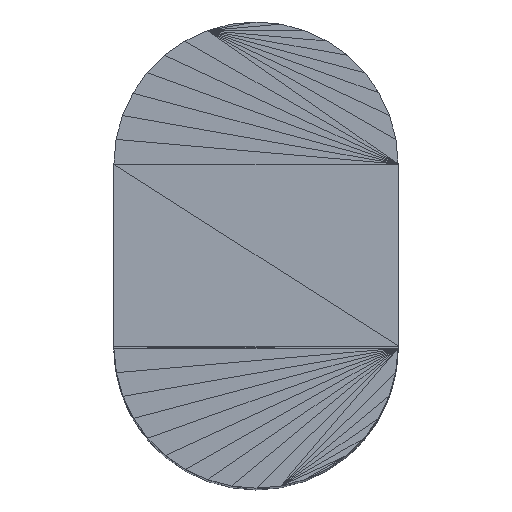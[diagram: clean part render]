
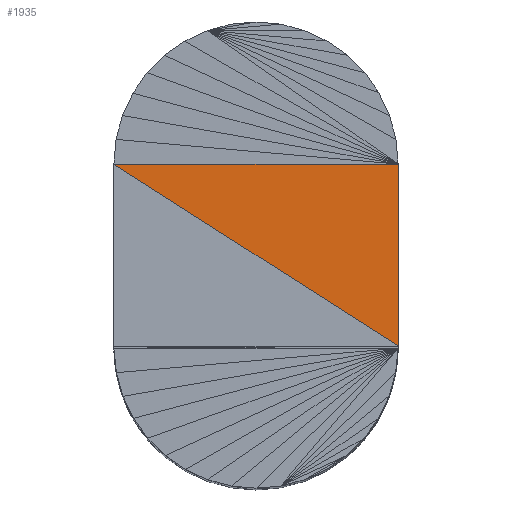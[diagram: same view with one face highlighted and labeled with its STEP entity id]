
A CAD part, top view. The second image highlights one B-rep face of the part: STEP entity #1935.
In plain terms, the highlighted planar face has unit normal (0, 0, 1).
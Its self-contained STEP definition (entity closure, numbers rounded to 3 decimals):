
#261 = VECTOR ( 'NONE', #16256, 1000. ) ;
#1079 = VERTEX_POINT ( 'NONE', #17094 ) ;
#1267 = CARTESIAN_POINT ( 'NONE',  ( 0., 0., 219.3 ) ) ;
#1935 = ADVANCED_FACE ( 'NONE', ( #3157 ), #8545, .T. ) ;
#2330 = CARTESIAN_POINT ( 'NONE',  ( 30., 47.167, 219.3 ) ) ;
#2712 = LINE ( 'NONE', #6773, #261 ) ;
#3023 = CARTESIAN_POINT ( 'NONE',  ( 30., 27.969, 219.3 ) ) ;
#3157 = FACE_OUTER_BOUND ( 'NONE', #10537, .T. ) ;
#3300 = LINE ( 'NONE', #9898, #7817 ) ;
#3985 = DIRECTION ( 'NONE',  ( 0., 0., 1. ) ) ;
#4790 = LINE ( 'NONE', #15415, #9837 ) ;
#5311 = DIRECTION ( 'NONE',  ( 1., 0., 0. ) ) ;
#5734 = EDGE_CURVE ( 'NONE', #10033, #10195, #3300, .T. ) ;
#6773 = CARTESIAN_POINT ( 'NONE',  ( 30., 47.167, 219.3 ) ) ;
#6809 = EDGE_CURVE ( 'NONE', #10033, #1079, #2712, .T. ) ;
#7473 = ORIENTED_EDGE ( 'NONE', *, *, #10235, .T. ) ;
#7817 = VECTOR ( 'NONE', #9988, 1000. ) ;
#8545 = PLANE ( 'NONE',  #17269 ) ;
#9802 = DIRECTION ( 'NONE',  ( 0.842, -0.539, 0. ) ) ;
#9837 = VECTOR ( 'NONE', #9802, 1000. ) ;
#9898 = CARTESIAN_POINT ( 'NONE',  ( 30., 47.167, 219.3 ) ) ;
#9988 = DIRECTION ( 'NONE',  ( 0., -1., 0. ) ) ;
#10033 = VERTEX_POINT ( 'NONE', #2330 ) ;
#10195 = VERTEX_POINT ( 'NONE', #3023 ) ;
#10235 = EDGE_CURVE ( 'NONE', #1079, #10195, #4790, .T. ) ;
#10537 = EDGE_LOOP ( 'NONE', ( #14608, #13373, #7473 ) ) ;
#13373 = ORIENTED_EDGE ( 'NONE', *, *, #6809, .T. ) ;
#14608 = ORIENTED_EDGE ( 'NONE', *, *, #5734, .F. ) ;
#15415 = CARTESIAN_POINT ( 'NONE',  ( 0., 47.167, 219.3 ) ) ;
#16256 = DIRECTION ( 'NONE',  ( -1., 0., 0. ) ) ;
#17094 = CARTESIAN_POINT ( 'NONE',  ( 0., 47.167, 219.3 ) ) ;
#17269 = AXIS2_PLACEMENT_3D ( 'NONE', #1267, #3985, #5311 ) ;
